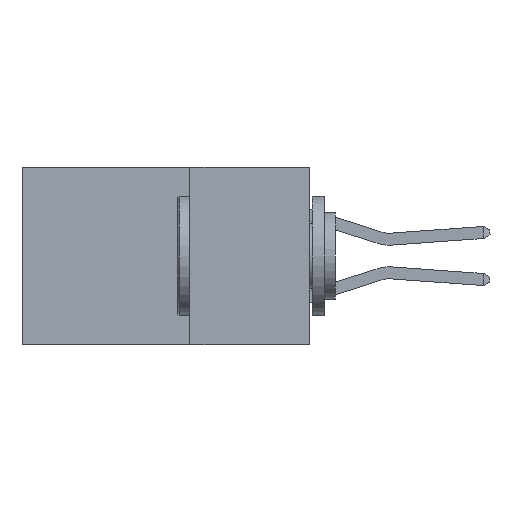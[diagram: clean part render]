
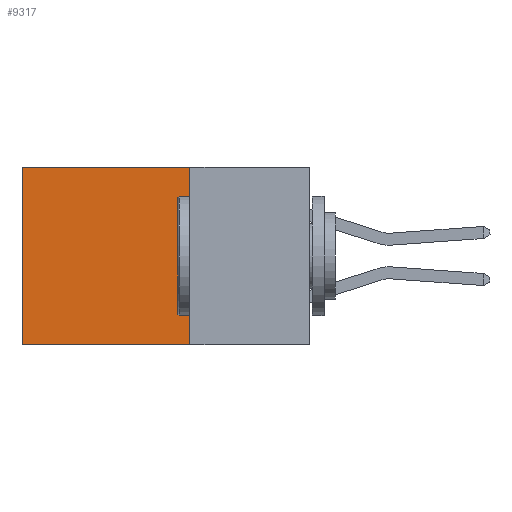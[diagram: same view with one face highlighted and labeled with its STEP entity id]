
A CAD part, left-side view. The second image highlights one B-rep face of the part: STEP entity #9317.
In plain terms, the highlighted planar face has unit normal (-1, 0, 0).
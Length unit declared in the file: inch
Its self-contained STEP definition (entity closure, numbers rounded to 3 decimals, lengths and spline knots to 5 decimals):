
#74 = DIRECTION ( 'NONE',  ( 0., 1., 0. ) ) ;
#121 = EDGE_CURVE ( 'NONE', #8542, #16685, #15315, .T. ) ;
#243 = CARTESIAN_POINT ( 'NONE',  ( 0.298, 0.25, 0. ) ) ;
#800 = DIRECTION ( 'NONE',  ( 0., 1., 0. ) ) ;
#999 = FACE_OUTER_BOUND ( 'NONE', #1517, .T. ) ;
#1227 = VECTOR ( 'NONE', #5744, 39.37008 ) ;
#1517 = EDGE_LOOP ( 'NONE', ( #13550, #4961, #14161, #13210 ) ) ;
#2022 = CARTESIAN_POINT ( 'NONE',  ( 0.298, 0.25, 0. ) ) ;
#2953 = VERTEX_POINT ( 'NONE', #14924 ) ;
#3080 = CARTESIAN_POINT ( 'NONE',  ( 0.298, 0.25, -0.37 ) ) ;
#3806 = VERTEX_POINT ( 'NONE', #8803 ) ;
#3818 = CARTESIAN_POINT ( 'NONE',  ( 0.298, 0.25, 0. ) ) ;
#4328 = VECTOR ( 'NONE', #15613, 39.37008 ) ;
#4498 = CARTESIAN_POINT ( 'NONE',  ( 0.298, 0.25, -0.37 ) ) ;
#4557 = LINE ( 'NONE', #243, #7694 ) ;
#4961 = ORIENTED_EDGE ( 'NONE', *, *, #5161, .F. ) ;
#5161 = EDGE_CURVE ( 'NONE', #16685, #2953, #15985, .T. ) ;
#5357 = VECTOR ( 'NONE', #800, 39.37008 ) ;
#5744 = DIRECTION ( 'NONE',  ( 0., 0., -1. ) ) ;
#6234 = DIRECTION ( 'NONE',  ( 1., 0., 0. ) ) ;
#6419 = AXIS2_PLACEMENT_3D ( 'NONE', #12815, #6234, #15534 ) ;
#6639 = EDGE_CURVE ( 'NONE', #8542, #3806, #4557, .T. ) ;
#7300 = EDGE_CURVE ( 'NONE', #3806, #2953, #11424, .T. ) ;
#7694 = VECTOR ( 'NONE', #74, 39.37008 ) ;
#8542 = VERTEX_POINT ( 'NONE', #2022 ) ;
#8803 = CARTESIAN_POINT ( 'NONE',  ( 0.298, 0.6, 0. ) ) ;
#9317 = ADVANCED_FACE ( 'NONE', ( #999 ), #14193, .F. ) ;
#11424 = LINE ( 'NONE', #15645, #4328 ) ;
#12815 = CARTESIAN_POINT ( 'NONE',  ( 0.298, 0.25, 0. ) ) ;
#13210 = ORIENTED_EDGE ( 'NONE', *, *, #6639, .T. ) ;
#13550 = ORIENTED_EDGE ( 'NONE', *, *, #7300, .T. ) ;
#14161 = ORIENTED_EDGE ( 'NONE', *, *, #121, .F. ) ;
#14193 = PLANE ( 'NONE',  #6419 ) ;
#14924 = CARTESIAN_POINT ( 'NONE',  ( 0.298, 0.6, -0.37 ) ) ;
#15315 = LINE ( 'NONE', #3818, #1227 ) ;
#15534 = DIRECTION ( 'NONE',  ( 0., 0., -1. ) ) ;
#15613 = DIRECTION ( 'NONE',  ( 0., 0., -1. ) ) ;
#15645 = CARTESIAN_POINT ( 'NONE',  ( 0.298, 0.6, 0. ) ) ;
#15985 = LINE ( 'NONE', #3080, #5357 ) ;
#16685 = VERTEX_POINT ( 'NONE', #4498 ) ;
